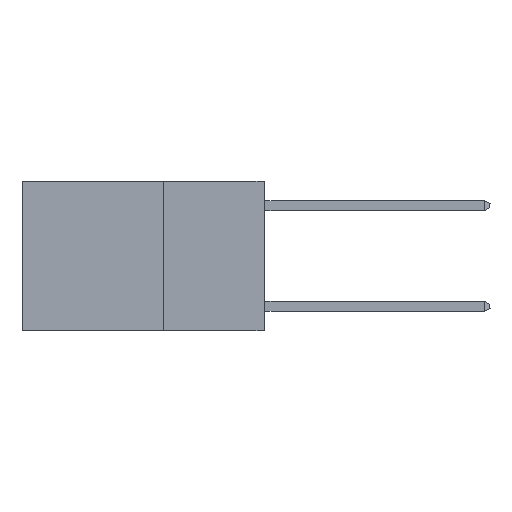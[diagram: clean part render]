
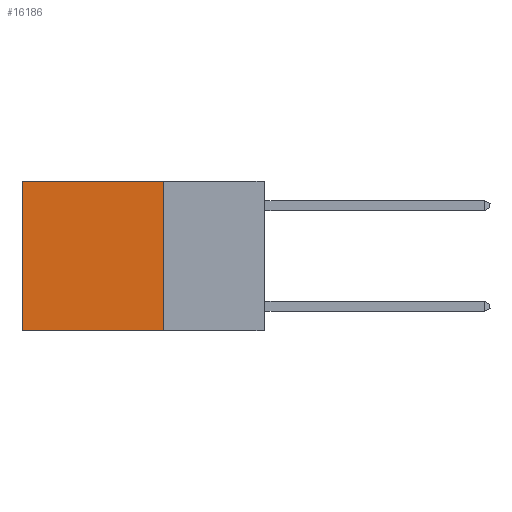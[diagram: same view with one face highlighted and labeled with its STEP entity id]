
A CAD part, left-side view. The second image highlights one B-rep face of the part: STEP entity #16186.
In plain terms, the highlighted planar face has unit normal (-1, 0, 0).
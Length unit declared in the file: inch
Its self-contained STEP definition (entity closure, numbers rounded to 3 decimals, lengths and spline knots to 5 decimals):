
#142 = PLANE ( 'NONE',  #13811 ) ;
#339 = FACE_OUTER_BOUND ( 'NONE', #16157, .T. ) ;
#1053 = LINE ( 'NONE', #16806, #5500 ) ;
#2932 = CARTESIAN_POINT ( 'NONE',  ( 0.2625, 0.25, -0.37 ) ) ;
#3053 = VECTOR ( 'NONE', #16838, 39.37008 ) ;
#3252 = CARTESIAN_POINT ( 'NONE',  ( 0.2625, 0.25, 0. ) ) ;
#3300 = ORIENTED_EDGE ( 'NONE', *, *, #14514, .T. ) ;
#3345 = CARTESIAN_POINT ( 'NONE',  ( 0.2625, 0.6, -0.37 ) ) ;
#4484 = CARTESIAN_POINT ( 'NONE',  ( 0.2625, 0.25, 0. ) ) ;
#5500 = VECTOR ( 'NONE', #7409, 39.37008 ) ;
#6155 = VERTEX_POINT ( 'NONE', #9521 ) ;
#6924 = CARTESIAN_POINT ( 'NONE',  ( 0.2625, 0.25, 0. ) ) ;
#7409 = DIRECTION ( 'NONE',  ( 0., 0., -1. ) ) ;
#7577 = VERTEX_POINT ( 'NONE', #2932 ) ;
#8333 = DIRECTION ( 'NONE',  ( 0., 1., 0. ) ) ;
#9521 = CARTESIAN_POINT ( 'NONE',  ( 0.2625, 0.6, 0. ) ) ;
#10475 = LINE ( 'NONE', #11645, #3053 ) ;
#11359 = VERTEX_POINT ( 'NONE', #3345 ) ;
#11645 = CARTESIAN_POINT ( 'NONE',  ( 0.2625, 0.25, 0. ) ) ;
#12251 = VERTEX_POINT ( 'NONE', #6924 ) ;
#12456 = LINE ( 'NONE', #4484, #18750 ) ;
#13811 = AXIS2_PLACEMENT_3D ( 'NONE', #3252, #14757, #15997 ) ;
#14514 = EDGE_CURVE ( 'NONE', #12251, #6155, #10475, .T. ) ;
#14631 = CARTESIAN_POINT ( 'NONE',  ( 0.2625, 0.25, -0.37 ) ) ;
#14757 = DIRECTION ( 'NONE',  ( 1., 0., 0. ) ) ;
#14997 = EDGE_CURVE ( 'NONE', #12251, #7577, #12456, .T. ) ;
#15461 = ORIENTED_EDGE ( 'NONE', *, *, #14997, .F. ) ;
#15666 = ORIENTED_EDGE ( 'NONE', *, *, #18579, .F. ) ;
#15997 = DIRECTION ( 'NONE',  ( 0., 0., -1. ) ) ;
#16157 = EDGE_LOOP ( 'NONE', ( #19759, #15666, #15461, #3300 ) ) ;
#16186 = ADVANCED_FACE ( 'NONE', ( #339 ), #142, .F. ) ;
#16806 = CARTESIAN_POINT ( 'NONE',  ( 0.2625, 0.6, 0. ) ) ;
#16838 = DIRECTION ( 'NONE',  ( 0., 1., 0. ) ) ;
#17226 = DIRECTION ( 'NONE',  ( 0., 0., -1. ) ) ;
#18305 = EDGE_CURVE ( 'NONE', #6155, #11359, #1053, .T. ) ;
#18579 = EDGE_CURVE ( 'NONE', #7577, #11359, #19522, .T. ) ;
#18750 = VECTOR ( 'NONE', #17226, 39.37008 ) ;
#19522 = LINE ( 'NONE', #14631, #19860 ) ;
#19759 = ORIENTED_EDGE ( 'NONE', *, *, #18305, .T. ) ;
#19860 = VECTOR ( 'NONE', #8333, 39.37008 ) ;
